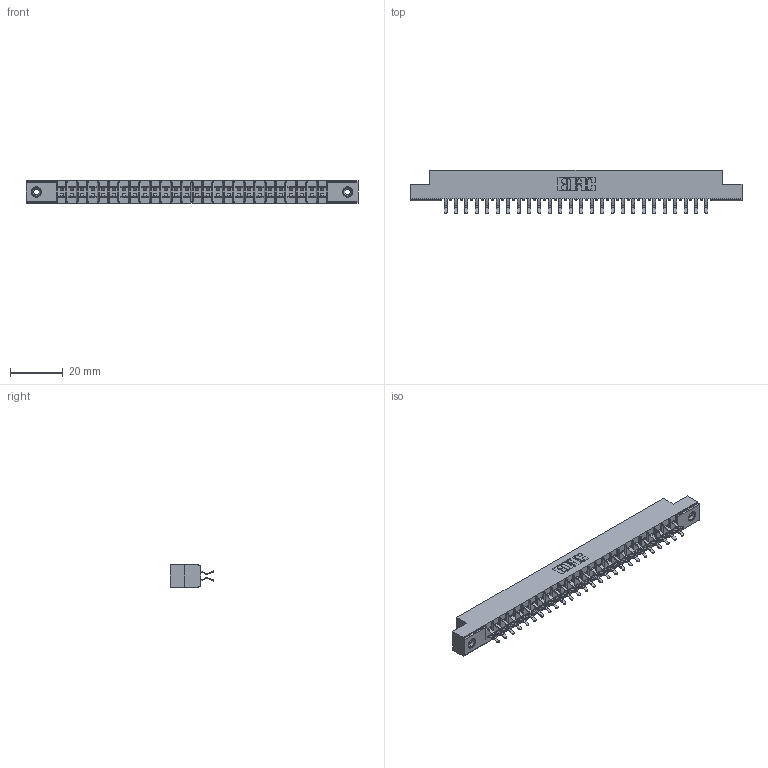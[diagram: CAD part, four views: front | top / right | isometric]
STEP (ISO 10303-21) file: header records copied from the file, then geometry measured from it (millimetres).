
FILE_DESCRIPTION (( 'STEP AP203' ), '1' );
FILE_NAME ('355-052-556-208.STEP', '2019-09-11T16:41:23', ( '' ), ( '' ), 'SwSTEP 2.0', 'SolidWorks 2016', '' );
FILE_SCHEMA (( 'CONFIG_CONTROL_DESIGN' ));
Length unit declared in the file: inch
Products named in the file (4): 355-052-556-208; 345-250-001_345-250-003-102; 305-290-001_556; 305 Part_.156 Dia
Assembly tree (55 placements, depth 2):
  355-052-556-208
    305 Part_.156 Dia
    305-290-001_556  x52
    345-250-001_345-250-003-102  x2
Bounding box: 126.03 x 16.64 x 8.71 mm (x, y, z)
Volume: 7880 mm3; surface area: 15168.2 mm2
Topology: 55 solids, 55 shells, 3088 faces, 8850 edges, 5752 vertices
Faces by surface type: plane 1712, cylinder 1256, sphere 104, cone 12, torus 4
Entity records: 31506 total; most frequent: CARTESIAN_POINT 5199, ORIENTED_EDGE 5152, DIRECTION 5056, EDGE_CURVE 2576, VECTOR 2058, LINE 2058, VERTEX_POINT 1642, AXIS2_PLACEMENT_3D 1499
